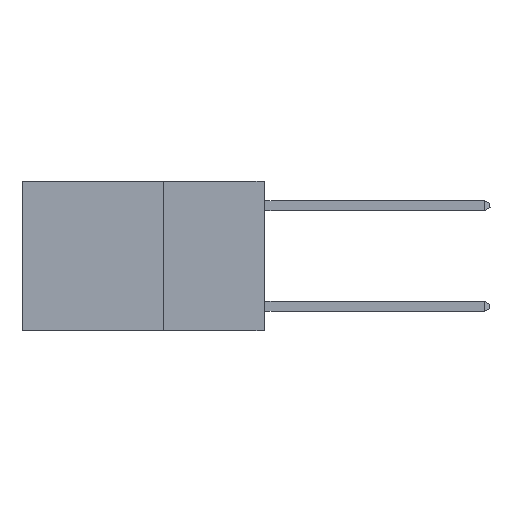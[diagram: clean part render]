
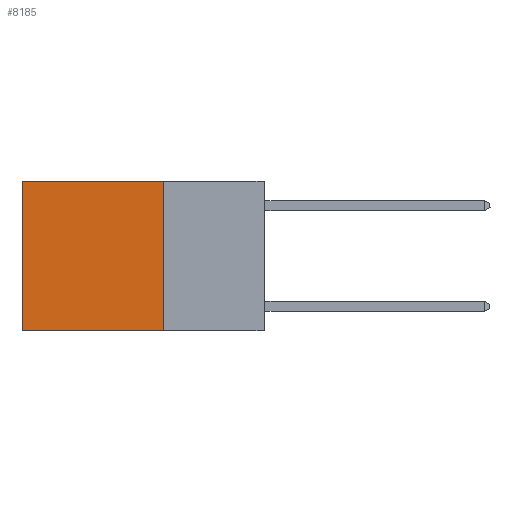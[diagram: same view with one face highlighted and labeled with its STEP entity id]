
A CAD part, left-side view. The second image highlights one B-rep face of the part: STEP entity #8185.
In plain terms, the highlighted planar face has unit normal (-1, 0, 0).
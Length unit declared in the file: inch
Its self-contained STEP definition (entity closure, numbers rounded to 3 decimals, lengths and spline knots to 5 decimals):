
#258 = CARTESIAN_POINT ( 'NONE',  ( 0.2625, 0.25, -0.37 ) ) ;
#362 = CARTESIAN_POINT ( 'NONE',  ( 0.2625, 0.6, -0.37 ) ) ;
#455 = CARTESIAN_POINT ( 'NONE',  ( 0.2625, 0.25, 0. ) ) ;
#718 = CARTESIAN_POINT ( 'NONE',  ( 0.2625, 0.25, 0. ) ) ;
#2615 = VERTEX_POINT ( 'NONE', #258 ) ;
#3098 = EDGE_CURVE ( 'NONE', #2615, #14463, #9514, .T. ) ;
#3945 = LINE ( 'NONE', #6417, #4272 ) ;
#4121 = ORIENTED_EDGE ( 'NONE', *, *, #25718, .F. ) ;
#4269 = DIRECTION ( 'NONE',  ( 0., 0., -1. ) ) ;
#4272 = VECTOR ( 'NONE', #4269, 39.37008 ) ;
#4619 = DIRECTION ( 'NONE',  ( 0., 0., -1. ) ) ;
#5103 = PLANE ( 'NONE',  #15371 ) ;
#5166 = ORIENTED_EDGE ( 'NONE', *, *, #6844, .T. ) ;
#6417 = CARTESIAN_POINT ( 'NONE',  ( 0.2625, 0.6, 0. ) ) ;
#6844 = EDGE_CURVE ( 'NONE', #23179, #25581, #25118, .T. ) ;
#7843 = VECTOR ( 'NONE', #4619, 39.37008 ) ;
#8185 = ADVANCED_FACE ( 'NONE', ( #9698 ), #5103, .F. ) ;
#9126 = DIRECTION ( 'NONE',  ( 0., 1., 0. ) ) ;
#9514 = LINE ( 'NONE', #15625, #22193 ) ;
#9698 = FACE_OUTER_BOUND ( 'NONE', #19670, .T. ) ;
#11709 = DIRECTION ( 'NONE',  ( 0., 0., -1. ) ) ;
#14463 = VERTEX_POINT ( 'NONE', #362 ) ;
#15371 = AXIS2_PLACEMENT_3D ( 'NONE', #23001, #20661, #11709 ) ;
#15625 = CARTESIAN_POINT ( 'NONE',  ( 0.2625, 0.25, -0.37 ) ) ;
#18107 = CARTESIAN_POINT ( 'NONE',  ( 0.2625, 0.25, 0. ) ) ;
#19246 = EDGE_CURVE ( 'NONE', #25581, #14463, #3945, .T. ) ;
#19670 = EDGE_LOOP ( 'NONE', ( #24607, #24952, #4121, #5166 ) ) ;
#19835 = LINE ( 'NONE', #18107, #7843 ) ;
#20661 = DIRECTION ( 'NONE',  ( 1., 0., 0. ) ) ;
#20854 = DIRECTION ( 'NONE',  ( 0., 1., 0. ) ) ;
#22193 = VECTOR ( 'NONE', #9126, 39.37008 ) ;
#23001 = CARTESIAN_POINT ( 'NONE',  ( 0.2625, 0.25, 0. ) ) ;
#23179 = VERTEX_POINT ( 'NONE', #455 ) ;
#24607 = ORIENTED_EDGE ( 'NONE', *, *, #19246, .T. ) ;
#24952 = ORIENTED_EDGE ( 'NONE', *, *, #3098, .F. ) ;
#25118 = LINE ( 'NONE', #718, #25281 ) ;
#25281 = VECTOR ( 'NONE', #20854, 39.37008 ) ;
#25581 = VERTEX_POINT ( 'NONE', #28957 ) ;
#25718 = EDGE_CURVE ( 'NONE', #23179, #2615, #19835, .T. ) ;
#28957 = CARTESIAN_POINT ( 'NONE',  ( 0.2625, 0.6, 0. ) ) ;
